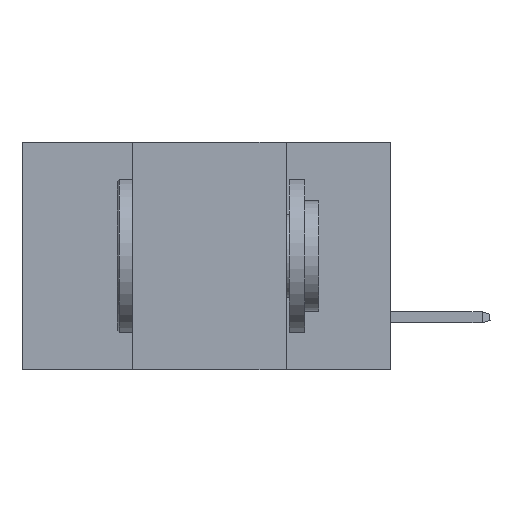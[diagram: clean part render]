
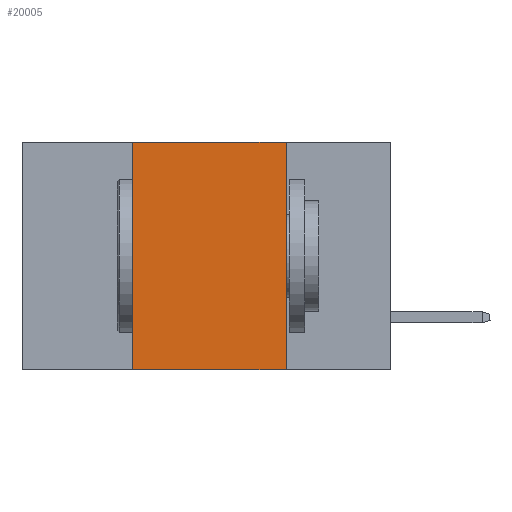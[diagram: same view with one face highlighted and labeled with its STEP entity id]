
A CAD part, left-side view. The second image highlights one B-rep face of the part: STEP entity #20005.
In plain terms, the highlighted planar face has unit normal (-1, 0, 0).
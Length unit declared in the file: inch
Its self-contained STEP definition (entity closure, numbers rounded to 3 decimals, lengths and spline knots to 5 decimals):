
#1059 = DIRECTION ( 'NONE',  ( 0., 0., -1. ) ) ;
#1483 = EDGE_LOOP ( 'NONE', ( #8346, #23078, #20216, #7756 ) ) ;
#2462 = CARTESIAN_POINT ( 'NONE',  ( 0., 0.42, 0. ) ) ;
#2761 = VECTOR ( 'NONE', #4387, 39.37008 ) ;
#4387 = DIRECTION ( 'NONE',  ( 0., -1., 0. ) ) ;
#4975 = DIRECTION ( 'NONE',  ( 0., 0., 1. ) ) ;
#5621 = VERTEX_POINT ( 'NONE', #12251 ) ;
#6106 = CARTESIAN_POINT ( 'NONE',  ( 0., 0.17, 0. ) ) ;
#6416 = VECTOR ( 'NONE', #4975, 39.37008 ) ;
#6860 = CARTESIAN_POINT ( 'NONE',  ( 0., 0.6, 0. ) ) ;
#7136 = EDGE_CURVE ( 'NONE', #5621, #14412, #23030, .T. ) ;
#7513 = AXIS2_PLACEMENT_3D ( 'NONE', #6860, #8781, #1059 ) ;
#7756 = ORIENTED_EDGE ( 'NONE', *, *, #9959, .T. ) ;
#8346 = ORIENTED_EDGE ( 'NONE', *, *, #14958, .F. ) ;
#8781 = DIRECTION ( 'NONE',  ( 1., 0., 0. ) ) ;
#9520 = VECTOR ( 'NONE', #17901, 39.37008 ) ;
#9959 = EDGE_CURVE ( 'NONE', #5621, #21132, #22276, .T. ) ;
#10163 = FACE_OUTER_BOUND ( 'NONE', #1483, .T. ) ;
#10205 = CARTESIAN_POINT ( 'NONE',  ( 0., 0.17, 0. ) ) ;
#10550 = CARTESIAN_POINT ( 'NONE',  ( 0., 0.6, -0.37 ) ) ;
#12251 = CARTESIAN_POINT ( 'NONE',  ( 0., 0.42, -0.37 ) ) ;
#12997 = CARTESIAN_POINT ( 'NONE',  ( 0., 0.42, 0. ) ) ;
#14412 = VERTEX_POINT ( 'NONE', #2462 ) ;
#14945 = VERTEX_POINT ( 'NONE', #10205 ) ;
#14958 = EDGE_CURVE ( 'NONE', #14945, #21132, #19210, .T. ) ;
#15940 = CARTESIAN_POINT ( 'NONE',  ( 0., 0.6, 0. ) ) ;
#17901 = DIRECTION ( 'NONE',  ( 0., 0., -1. ) ) ;
#19210 = LINE ( 'NONE', #6106, #9520 ) ;
#20005 = ADVANCED_FACE ( 'NONE', ( #10163 ), #24164, .F. ) ;
#20216 = ORIENTED_EDGE ( 'NONE', *, *, #7136, .F. ) ;
#20659 = LINE ( 'NONE', #15940, #2761 ) ;
#21032 = CARTESIAN_POINT ( 'NONE',  ( 0., 0.17, -0.37 ) ) ;
#21132 = VERTEX_POINT ( 'NONE', #21032 ) ;
#22276 = LINE ( 'NONE', #10550, #23178 ) ;
#23030 = LINE ( 'NONE', #12997, #6416 ) ;
#23078 = ORIENTED_EDGE ( 'NONE', *, *, #23255, .F. ) ;
#23178 = VECTOR ( 'NONE', #24187, 39.37008 ) ;
#23255 = EDGE_CURVE ( 'NONE', #14412, #14945, #20659, .T. ) ;
#24164 = PLANE ( 'NONE',  #7513 ) ;
#24187 = DIRECTION ( 'NONE',  ( 0., -1., 0. ) ) ;
